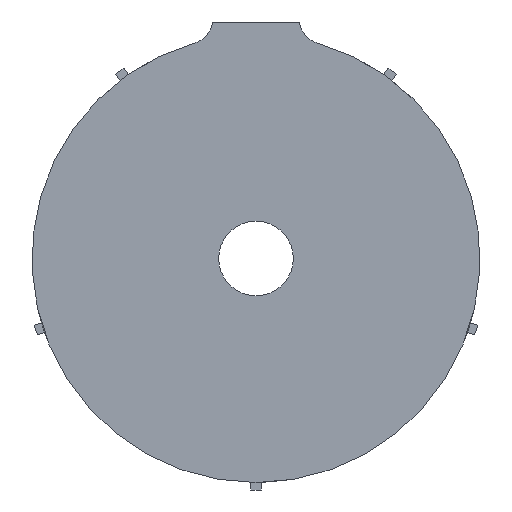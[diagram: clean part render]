
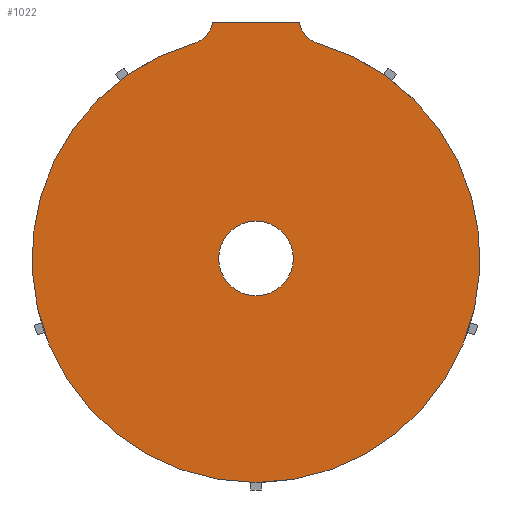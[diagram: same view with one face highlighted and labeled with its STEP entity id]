
A CAD part, front view. The second image highlights one B-rep face of the part: STEP entity #1022.
In plain terms, the highlighted planar face has unit normal (0, -1, 0).
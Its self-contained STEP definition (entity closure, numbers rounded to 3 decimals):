
#3 = DIRECTION ( 'NONE',  ( 0., 0., 1. ) ) ;
#45 = EDGE_CURVE ( 'NONE', #3062, #1717, #528, .T. ) ;
#130 = DIRECTION ( 'NONE',  ( 0., 1., 0. ) ) ;
#153 = CARTESIAN_POINT ( 'NONE',  ( 0., 0., 0. ) ) ;
#210 = FACE_OUTER_BOUND ( 'NONE', #1134, .T. ) ;
#237 = DIRECTION ( 'NONE',  ( 0., 1., 0. ) ) ;
#284 = EDGE_CURVE ( 'NONE', #649, #2128, #1681, .T. ) ;
#323 = VERTEX_POINT ( 'NONE', #2483 ) ;
#399 = CARTESIAN_POINT ( 'NONE',  ( 0., 0., 0. ) ) ;
#416 = DIRECTION ( 'NONE',  ( 0., 0., 1. ) ) ;
#417 = DIRECTION ( 'NONE',  ( 1., 0., 0. ) ) ;
#468 = ORIENTED_EDGE ( 'NONE', *, *, #284, .T. ) ;
#528 = CIRCLE ( 'NONE', #2733, 15. ) ;
#546 = CARTESIAN_POINT ( 'NONE',  ( -17.5, 0., 95. ) ) ;
#571 = DIRECTION ( 'NONE',  ( 0., 1., 0. ) ) ;
#649 = VERTEX_POINT ( 'NONE', #546 ) ;
#652 = DIRECTION ( 'NONE',  ( 0., 0., 1. ) ) ;
#771 = AXIS2_PLACEMENT_3D ( 'NONE', #2120, #571, #2383 ) ;
#851 = CARTESIAN_POINT ( 'NONE',  ( 0., 0., 15. ) ) ;
#919 = ORIENTED_EDGE ( 'NONE', *, *, #45, .T. ) ;
#1022 = ADVANCED_FACE ( 'NONE', ( #210, #1581 ), #1436, .F. ) ;
#1134 = EDGE_LOOP ( 'NONE', ( #2302, #2382, #1990, #468, #2535 ) ) ;
#1188 = CARTESIAN_POINT ( 'NONE',  ( 17.5, 0., 95. ) ) ;
#1229 = VECTOR ( 'NONE', #417, 1000. ) ;
#1270 = CARTESIAN_POINT ( 'NONE',  ( 27.432, 0., 96.164 ) ) ;
#1345 = VERTEX_POINT ( 'NONE', #2900 ) ;
#1379 = CIRCLE ( 'NONE', #2621, 90. ) ;
#1428 = CARTESIAN_POINT ( 'NONE',  ( 0., 0., -15. ) ) ;
#1436 = PLANE ( 'NONE',  #3094 ) ;
#1501 = EDGE_CURVE ( 'NONE', #323, #2128, #1379, .T. ) ;
#1527 = DIRECTION ( 'NONE',  ( 0., 0., 1. ) ) ;
#1553 = EDGE_CURVE ( 'NONE', #649, #2372, #1907, .T. ) ;
#1569 = CARTESIAN_POINT ( 'NONE',  ( -24.689, 0., 86.547 ) ) ;
#1581 = FACE_BOUND ( 'NONE', #3247, .T. ) ;
#1673 = CARTESIAN_POINT ( 'NONE',  ( -27.432, 0., 96.164 ) ) ;
#1681 = CIRCLE ( 'NONE', #1818, 10. ) ;
#1717 = VERTEX_POINT ( 'NONE', #851 ) ;
#1780 = CARTESIAN_POINT ( 'NONE',  ( 0., 0., 0. ) ) ;
#1818 = AXIS2_PLACEMENT_3D ( 'NONE', #1673, #130, #1933 ) ;
#1907 = LINE ( 'NONE', #1188, #1229 ) ;
#1912 = CARTESIAN_POINT ( 'NONE',  ( 17.5, 0., 95. ) ) ;
#1918 = DIRECTION ( 'NONE',  ( 0., 1., 0. ) ) ;
#1933 = DIRECTION ( 'NONE',  ( 0., 0., 1. ) ) ;
#1950 = DIRECTION ( 'NONE',  ( 0., 1., 0. ) ) ;
#1990 = ORIENTED_EDGE ( 'NONE', *, *, #1553, .F. ) ;
#2034 = DIRECTION ( 'NONE',  ( 0., 0., 1. ) ) ;
#2120 = CARTESIAN_POINT ( 'NONE',  ( 0., 0., 0. ) ) ;
#2128 = VERTEX_POINT ( 'NONE', #1569 ) ;
#2192 = EDGE_CURVE ( 'NONE', #1717, #3062, #3114, .T. ) ;
#2207 = DIRECTION ( 'NONE',  ( 0., 1., 0. ) ) ;
#2302 = ORIENTED_EDGE ( 'NONE', *, *, #2644, .F. ) ;
#2333 = ORIENTED_EDGE ( 'NONE', *, *, #2192, .T. ) ;
#2372 = VERTEX_POINT ( 'NONE', #1912 ) ;
#2382 = ORIENTED_EDGE ( 'NONE', *, *, #2651, .T. ) ;
#2383 = DIRECTION ( 'NONE',  ( 0., 0., 1. ) ) ;
#2434 = CIRCLE ( 'NONE', #3110, 10. ) ;
#2483 = CARTESIAN_POINT ( 'NONE',  ( 0., 0., -90. ) ) ;
#2535 = ORIENTED_EDGE ( 'NONE', *, *, #1501, .F. ) ;
#2621 = AXIS2_PLACEMENT_3D ( 'NONE', #399, #2207, #652 ) ;
#2644 = EDGE_CURVE ( 'NONE', #1345, #323, #3191, .T. ) ;
#2651 = EDGE_CURVE ( 'NONE', #1345, #2372, #2434, .T. ) ;
#2733 = AXIS2_PLACEMENT_3D ( 'NONE', #2942, #1918, #3 ) ;
#2900 = CARTESIAN_POINT ( 'NONE',  ( 24.689, 0., 86.547 ) ) ;
#2942 = CARTESIAN_POINT ( 'NONE',  ( 0., 0., 0. ) ) ;
#3062 = VERTEX_POINT ( 'NONE', #1428 ) ;
#3067 = DIRECTION ( 'NONE',  ( 0., 1., 0. ) ) ;
#3094 = AXIS2_PLACEMENT_3D ( 'NONE', #153, #1950, #416 ) ;
#3110 = AXIS2_PLACEMENT_3D ( 'NONE', #1270, #3067, #1527 ) ;
#3114 = CIRCLE ( 'NONE', #771, 15. ) ;
#3191 = CIRCLE ( 'NONE', #3278, 90. ) ;
#3247 = EDGE_LOOP ( 'NONE', ( #919, #2333 ) ) ;
#3278 = AXIS2_PLACEMENT_3D ( 'NONE', #1780, #237, #2034 ) ;
